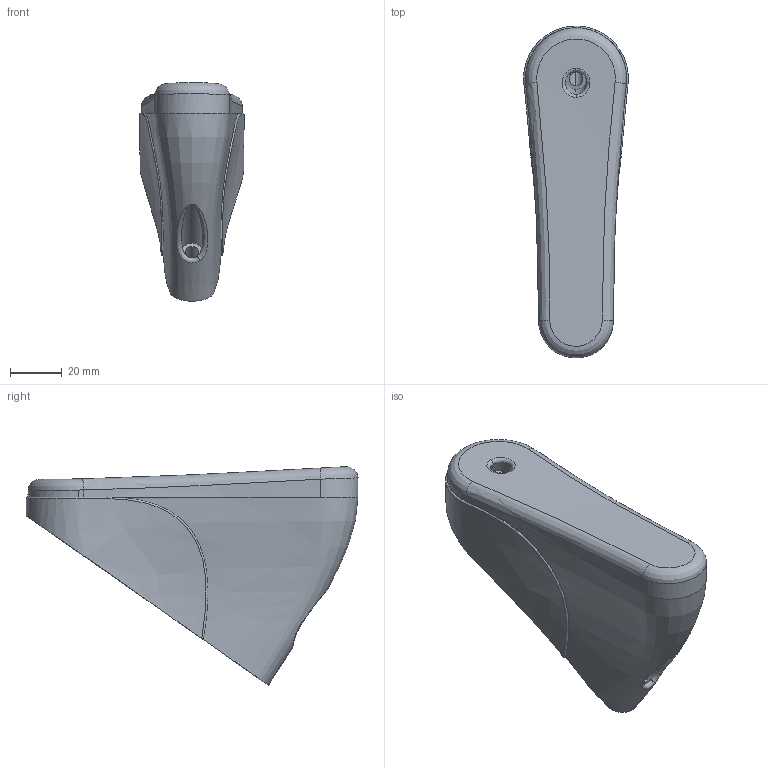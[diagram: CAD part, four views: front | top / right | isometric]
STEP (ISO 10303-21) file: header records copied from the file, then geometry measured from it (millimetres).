
FILE_DESCRIPTION (( 'STEP AP203' ), '1' );
FILE_NAME ('Orca Stock Butt V5.3.STEP', '2023-01-20T23:43:50', ( '' ), ( '' ), 'SwSTEP 2.0', 'SolidWorks 2021', '' );
FILE_SCHEMA (( 'CONFIG_CONTROL_DESIGN' ));
Length unit declared in the file: inch
Products named in the file (1): Orca Stock Butt V5.3
Bounding box: 40.6 x 128.78 x 84.75 mm (x, y, z)
Volume: 171416.8 mm3; surface area: 22316.5 mm2
Topology: 1 solids, 1 shells, 38 faces, 92 edges, 59 vertices
Faces by surface type: bspline 19, cylinder 14, plane 5
Entity records: 19362 total; most frequent: CARTESIAN_POINT 18530, ORIENTED_EDGE 184, DIRECTION 108, EDGE_CURVE 92, VERTEX_POINT 59, B_SPLINE_CURVE_WITH_KNOTS 45, AXIS2_PLACEMENT_3D 45, EDGE_LOOP 45
